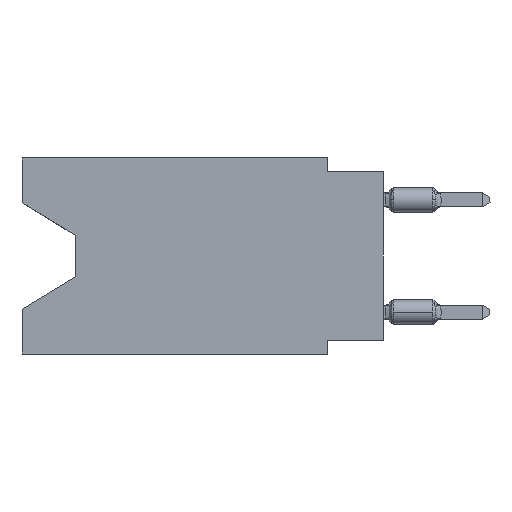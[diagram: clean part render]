
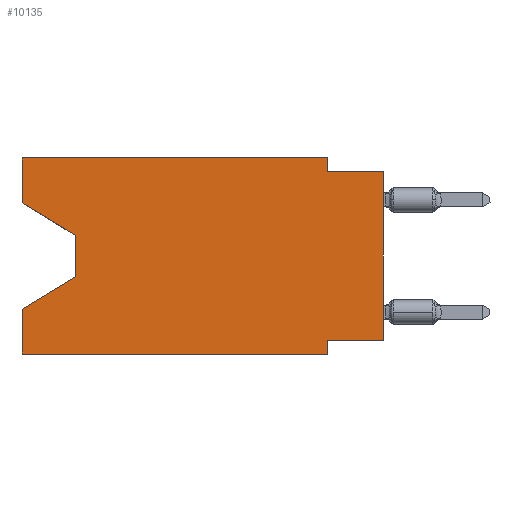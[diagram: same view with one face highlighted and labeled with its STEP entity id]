
A CAD part, left-side view. The second image highlights one B-rep face of the part: STEP entity #10135.
In plain terms, the highlighted planar face has unit normal (-1, 0, 0).
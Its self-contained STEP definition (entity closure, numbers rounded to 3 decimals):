
#88 = CARTESIAN_POINT ( 'NONE',  ( 0., 2.54, 0. ) ) ;
#90 = ORIENTED_EDGE ( 'NONE', *, *, #383, .F. ) ;
#363 = CARTESIAN_POINT ( 'NONE',  ( 0., 2.54, -8.89 ) ) ;
#383 = EDGE_CURVE ( 'NONE', #1259, #13749, #7289, .T. ) ;
#445 = VECTOR ( 'NONE', #3251, 1000. ) ;
#538 = CARTESIAN_POINT ( 'NONE',  ( 0., 16.383, 0. ) ) ;
#575 = EDGE_CURVE ( 'NONE', #7216, #1259, #4998, .T. ) ;
#580 = VERTEX_POINT ( 'NONE', #11867 ) ;
#613 = ORIENTED_EDGE ( 'NONE', *, *, #10217, .F. ) ;
#785 = CARTESIAN_POINT ( 'NONE',  ( 0., 0., -8.255 ) ) ;
#1043 = CARTESIAN_POINT ( 'NONE',  ( 0., 16.383, -6.852 ) ) ;
#1116 = CARTESIAN_POINT ( 'NONE',  ( 0., 2.54, -0.635 ) ) ;
#1183 = DIRECTION ( 'NONE',  ( 0., 1., 0. ) ) ;
#1259 = VERTEX_POINT ( 'NONE', #1116 ) ;
#1293 = CARTESIAN_POINT ( 'NONE',  ( 0., 16.383, 0. ) ) ;
#1424 = CARTESIAN_POINT ( 'NONE',  ( 0., 0., -0.635 ) ) ;
#1466 = CARTESIAN_POINT ( 'NONE',  ( 0., 16.383, 0. ) ) ;
#1508 = ORIENTED_EDGE ( 'NONE', *, *, #11593, .T. ) ;
#1632 = VERTEX_POINT ( 'NONE', #13799 ) ;
#1838 = DIRECTION ( 'NONE',  ( 0., -0.855, -0.519 ) ) ;
#2216 = DIRECTION ( 'NONE',  ( 0., 0., 1. ) ) ;
#2292 = VECTOR ( 'NONE', #1838, 1000. ) ;
#2397 = EDGE_CURVE ( 'NONE', #14881, #13749, #8217, .T. ) ;
#2589 = DIRECTION ( 'NONE',  ( 0., 0., 1. ) ) ;
#2637 = ORIENTED_EDGE ( 'NONE', *, *, #4922, .T. ) ;
#2769 = LINE ( 'NONE', #14312, #3633 ) ;
#3251 = DIRECTION ( 'NONE',  ( 0., 0., -1. ) ) ;
#3520 = DIRECTION ( 'NONE',  ( 0., 0.855, -0.519 ) ) ;
#3633 = VECTOR ( 'NONE', #10937, 1000. ) ;
#3734 = CARTESIAN_POINT ( 'NONE',  ( 0., 2.54, -8.255 ) ) ;
#3775 = LINE ( 'NONE', #7094, #12462 ) ;
#4333 = AXIS2_PLACEMENT_3D ( 'NONE', #1466, #6169, #14077 ) ;
#4382 = VECTOR ( 'NONE', #8953, 1000. ) ;
#4697 = PLANE ( 'NONE',  #4333 ) ;
#4922 = EDGE_CURVE ( 'NONE', #1632, #12142, #12393, .T. ) ;
#4931 = DIRECTION ( 'NONE',  ( 0., 0., -1. ) ) ;
#4998 = LINE ( 'NONE', #12938, #6596 ) ;
#5008 = CARTESIAN_POINT ( 'NONE',  ( 0., 16.383, 0. ) ) ;
#5325 = VERTEX_POINT ( 'NONE', #13582 ) ;
#5472 = ORIENTED_EDGE ( 'NONE', *, *, #575, .F. ) ;
#5498 = ORIENTED_EDGE ( 'NONE', *, *, #14538, .F. ) ;
#5844 = VECTOR ( 'NONE', #6479, 1000. ) ;
#6046 = VECTOR ( 'NONE', #3520, 1000. ) ;
#6051 = VECTOR ( 'NONE', #2216, 1000. ) ;
#6169 = DIRECTION ( 'NONE',  ( 1., 0., 0. ) ) ;
#6348 = EDGE_CURVE ( 'NONE', #11381, #14170, #14057, .T. ) ;
#6479 = DIRECTION ( 'NONE',  ( 0., 0., 1. ) ) ;
#6536 = ORIENTED_EDGE ( 'NONE', *, *, #8266, .F. ) ;
#6596 = VECTOR ( 'NONE', #4931, 1000. ) ;
#7094 = CARTESIAN_POINT ( 'NONE',  ( 0., 16.383, -8.89 ) ) ;
#7147 = CARTESIAN_POINT ( 'NONE',  ( 0., 0., 0. ) ) ;
#7202 = CARTESIAN_POINT ( 'NONE',  ( 0., 0., -8.255 ) ) ;
#7216 = VERTEX_POINT ( 'NONE', #88 ) ;
#7289 = LINE ( 'NONE', #1424, #4382 ) ;
#7393 = VECTOR ( 'NONE', #2589, 1000. ) ;
#7413 = DIRECTION ( 'NONE',  ( 0., -1., 0. ) ) ;
#7427 = LINE ( 'NONE', #5008, #5844 ) ;
#7562 = VECTOR ( 'NONE', #7413, 1000. ) ;
#8069 = LINE ( 'NONE', #1293, #6051 ) ;
#8217 = LINE ( 'NONE', #7147, #7393 ) ;
#8252 = CARTESIAN_POINT ( 'NONE',  ( 0., 13.97, -3.505 ) ) ;
#8266 = EDGE_CURVE ( 'NONE', #14641, #10609, #13791, .T. ) ;
#8496 = EDGE_CURVE ( 'NONE', #1632, #580, #7427, .T. ) ;
#8631 = ORIENTED_EDGE ( 'NONE', *, *, #2397, .T. ) ;
#8953 = DIRECTION ( 'NONE',  ( 0., -1., 0. ) ) ;
#9255 = EDGE_CURVE ( 'NONE', #5325, #14170, #8069, .T. ) ;
#9643 = DIRECTION ( 'NONE',  ( 0., -1., 0. ) ) ;
#9867 = VECTOR ( 'NONE', #1183, 1000. ) ;
#10119 = EDGE_CURVE ( 'NONE', #5325, #10609, #3775, .T. ) ;
#10135 = ADVANCED_FACE ( 'NONE', ( #12016 ), #4697, .F. ) ;
#10217 = EDGE_CURVE ( 'NONE', #580, #7216, #12331, .T. ) ;
#10609 = VERTEX_POINT ( 'NONE', #363 ) ;
#10703 = ORIENTED_EDGE ( 'NONE', *, *, #9255, .F. ) ;
#10815 = CARTESIAN_POINT ( 'NONE',  ( 0., 13.97, -5.385 ) ) ;
#10937 = DIRECTION ( 'NONE',  ( 0., 0., -1. ) ) ;
#11055 = ORIENTED_EDGE ( 'NONE', *, *, #8496, .F. ) ;
#11166 = CARTESIAN_POINT ( 'NONE',  ( 0., 16.383, -2.038 ) ) ;
#11381 = VERTEX_POINT ( 'NONE', #10815 ) ;
#11420 = CARTESIAN_POINT ( 'NONE',  ( 0., 2.54, -8.89 ) ) ;
#11593 = EDGE_CURVE ( 'NONE', #12142, #11381, #2769, .T. ) ;
#11814 = LINE ( 'NONE', #7202, #9867 ) ;
#11867 = CARTESIAN_POINT ( 'NONE',  ( 0., 16.383, 0. ) ) ;
#12016 = FACE_OUTER_BOUND ( 'NONE', #13734, .T. ) ;
#12142 = VERTEX_POINT ( 'NONE', #8252 ) ;
#12331 = LINE ( 'NONE', #538, #7562 ) ;
#12393 = LINE ( 'NONE', #11166, #2292 ) ;
#12462 = VECTOR ( 'NONE', #9643, 1000. ) ;
#12694 = ORIENTED_EDGE ( 'NONE', *, *, #6348, .T. ) ;
#12938 = CARTESIAN_POINT ( 'NONE',  ( 0., 2.54, 0. ) ) ;
#13582 = CARTESIAN_POINT ( 'NONE',  ( 0., 16.383, -8.89 ) ) ;
#13734 = EDGE_LOOP ( 'NONE', ( #2637, #1508, #12694, #10703, #13806, #6536, #5498, #8631, #90, #5472, #613, #11055 ) ) ;
#13749 = VERTEX_POINT ( 'NONE', #14067 ) ;
#13791 = LINE ( 'NONE', #11420, #445 ) ;
#13799 = CARTESIAN_POINT ( 'NONE',  ( 0., 16.383, -2.038 ) ) ;
#13806 = ORIENTED_EDGE ( 'NONE', *, *, #10119, .T. ) ;
#13977 = CARTESIAN_POINT ( 'NONE',  ( 0., 13.97, -5.385 ) ) ;
#14057 = LINE ( 'NONE', #13977, #6046 ) ;
#14067 = CARTESIAN_POINT ( 'NONE',  ( 0., 0., -0.635 ) ) ;
#14077 = DIRECTION ( 'NONE',  ( 0., 0., -1. ) ) ;
#14170 = VERTEX_POINT ( 'NONE', #1043 ) ;
#14312 = CARTESIAN_POINT ( 'NONE',  ( 0., 13.97, -3.505 ) ) ;
#14538 = EDGE_CURVE ( 'NONE', #14881, #14641, #11814, .T. ) ;
#14641 = VERTEX_POINT ( 'NONE', #3734 ) ;
#14881 = VERTEX_POINT ( 'NONE', #785 ) ;
